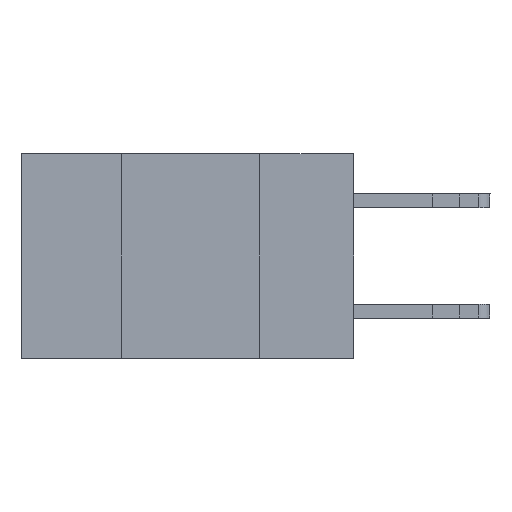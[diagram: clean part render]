
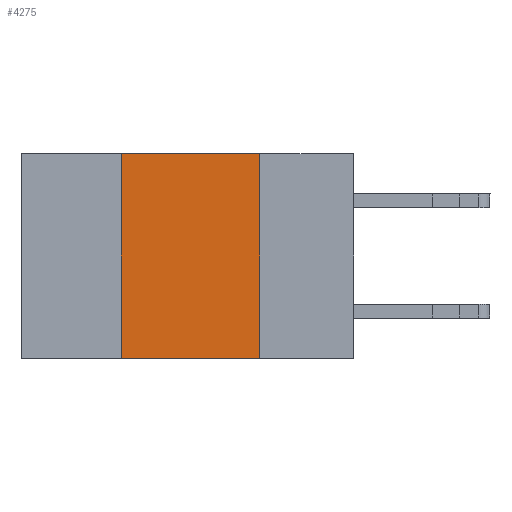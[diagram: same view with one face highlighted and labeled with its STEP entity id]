
A CAD part, left-side view. The second image highlights one B-rep face of the part: STEP entity #4275.
In plain terms, the highlighted planar face has unit normal (-1, 0, 0).
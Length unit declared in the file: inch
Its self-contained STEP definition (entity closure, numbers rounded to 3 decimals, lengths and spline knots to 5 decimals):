
#883 = ORIENTED_EDGE ( 'NONE', *, *, #5365, .F. ) ;
#1156 = ORIENTED_EDGE ( 'NONE', *, *, #22866, .F. ) ;
#2723 = DIRECTION ( 'NONE',  ( 0., 0., 1. ) ) ;
#2729 = FACE_OUTER_BOUND ( 'NONE', #11513, .T. ) ;
#2848 = VECTOR ( 'NONE', #17775, 39.37008 ) ;
#3101 = CARTESIAN_POINT ( 'NONE',  ( 0., 0.17, 0. ) ) ;
#3581 = LINE ( 'NONE', #20515, #13515 ) ;
#3616 = LINE ( 'NONE', #12615, #24141 ) ;
#3689 = ORIENTED_EDGE ( 'NONE', *, *, #4248, .F. ) ;
#3759 = AXIS2_PLACEMENT_3D ( 'NONE', #19809, #9913, #23813 ) ;
#4248 = EDGE_CURVE ( 'NONE', #11056, #11029, #4642, .T. ) ;
#4275 = ADVANCED_FACE ( 'NONE', ( #2729 ), #13782, .F. ) ;
#4642 = LINE ( 'NONE', #25683, #13284 ) ;
#5121 = CARTESIAN_POINT ( 'NONE',  ( 0., 0.42, 0. ) ) ;
#5365 = EDGE_CURVE ( 'NONE', #11644, #11056, #3616, .T. ) ;
#5485 = CARTESIAN_POINT ( 'NONE',  ( 0., 0.17, -0.37 ) ) ;
#6240 = VERTEX_POINT ( 'NONE', #5485 ) ;
#6894 = CARTESIAN_POINT ( 'NONE',  ( 0., 0.42, -0.37 ) ) ;
#8171 = LINE ( 'NONE', #15767, #2848 ) ;
#9832 = DIRECTION ( 'NONE',  ( 0., -1., 0. ) ) ;
#9913 = DIRECTION ( 'NONE',  ( 1., 0., 0. ) ) ;
#11029 = VERTEX_POINT ( 'NONE', #3101 ) ;
#11056 = VERTEX_POINT ( 'NONE', #5121 ) ;
#11513 = EDGE_LOOP ( 'NONE', ( #1156, #3689, #883, #17853 ) ) ;
#11644 = VERTEX_POINT ( 'NONE', #6894 ) ;
#12615 = CARTESIAN_POINT ( 'NONE',  ( 0., 0.42, 0. ) ) ;
#13284 = VECTOR ( 'NONE', #9832, 39.37008 ) ;
#13515 = VECTOR ( 'NONE', #22525, 39.37008 ) ;
#13782 = PLANE ( 'NONE',  #3759 ) ;
#15767 = CARTESIAN_POINT ( 'NONE',  ( 0., 0.6, -0.37 ) ) ;
#17775 = DIRECTION ( 'NONE',  ( 0., -1., 0. ) ) ;
#17853 = ORIENTED_EDGE ( 'NONE', *, *, #24688, .T. ) ;
#19809 = CARTESIAN_POINT ( 'NONE',  ( 0., 0.6, 0. ) ) ;
#20515 = CARTESIAN_POINT ( 'NONE',  ( 0., 0.17, 0. ) ) ;
#22525 = DIRECTION ( 'NONE',  ( 0., 0., -1. ) ) ;
#22866 = EDGE_CURVE ( 'NONE', #11029, #6240, #3581, .T. ) ;
#23813 = DIRECTION ( 'NONE',  ( 0., 0., -1. ) ) ;
#24141 = VECTOR ( 'NONE', #2723, 39.37008 ) ;
#24688 = EDGE_CURVE ( 'NONE', #11644, #6240, #8171, .T. ) ;
#25683 = CARTESIAN_POINT ( 'NONE',  ( 0., 0.6, 0. ) ) ;
